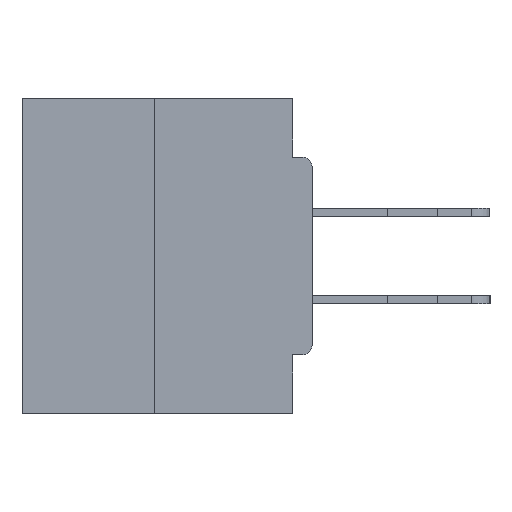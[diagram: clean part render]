
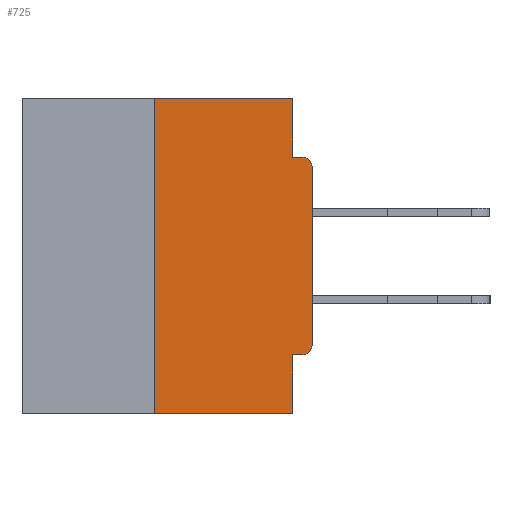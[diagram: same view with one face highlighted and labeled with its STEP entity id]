
A CAD part, left-side view. The second image highlights one B-rep face of the part: STEP entity #725.
In plain terms, the highlighted planar face has unit normal (-1, 0, 0).
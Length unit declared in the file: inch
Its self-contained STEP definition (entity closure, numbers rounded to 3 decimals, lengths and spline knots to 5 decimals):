
#447 = VECTOR ( 'NONE', #496, 39.37008 ) ;
#496 = DIRECTION ( 'NONE',  ( 0., 0., -1. ) ) ;
#539 = DIRECTION ( 'NONE',  ( 0., 0., 1. ) ) ;
#548 = VERTEX_POINT ( 'NONE', #23151 ) ;
#725 = ADVANCED_FACE ( 'NONE', ( #2220 ), #1923, .F. ) ;
#1036 = EDGE_CURVE ( 'NONE', #15112, #10786, #3096, .T. ) ;
#1923 = PLANE ( 'NONE',  #9730 ) ;
#2220 = FACE_OUTER_BOUND ( 'NONE', #24780, .T. ) ;
#2908 = DIRECTION ( 'NONE',  ( 0., -1., 0. ) ) ;
#3096 = LINE ( 'NONE', #11718, #33912 ) ;
#3262 = VECTOR ( 'NONE', #21967, 39.37008 ) ;
#4521 = EDGE_CURVE ( 'NONE', #15673, #548, #28752, .T. ) ;
#4667 = CARTESIAN_POINT ( 'NONE',  ( 0., 0.031, -0.4065 ) ) ;
#4798 = EDGE_CURVE ( 'NONE', #34067, #14897, #5996, .T. ) ;
#5551 = VECTOR ( 'NONE', #21708, 39.37008 ) ;
#5650 = ORIENTED_EDGE ( 'NONE', *, *, #13877, .F. ) ;
#5996 = LINE ( 'NONE', #7687, #3262 ) ;
#6161 = ORIENTED_EDGE ( 'NONE', *, *, #33916, .F. ) ;
#6210 = ORIENTED_EDGE ( 'NONE', *, *, #18368, .F. ) ;
#7275 = ORIENTED_EDGE ( 'NONE', *, *, #35363, .F. ) ;
#7687 = CARTESIAN_POINT ( 'NONE',  ( 0., 0.46, -0.5 ) ) ;
#7751 = CARTESIAN_POINT ( 'NONE',  ( 0., 0.015, -0.3915 ) ) ;
#8391 = DIRECTION ( 'NONE',  ( 0., -1., 0. ) ) ;
#9598 = VECTOR ( 'NONE', #8391, 39.37008 ) ;
#9730 = AXIS2_PLACEMENT_3D ( 'NONE', #25225, #10691, #13541 ) ;
#9937 = ORIENTED_EDGE ( 'NONE', *, *, #28549, .F. ) ;
#10206 = ORIENTED_EDGE ( 'NONE', *, *, #1036, .T. ) ;
#10496 = DIRECTION ( 'NONE',  ( -1., 0., 0. ) ) ;
#10594 = VERTEX_POINT ( 'NONE', #4667 ) ;
#10691 = DIRECTION ( 'NONE',  ( 1., 0., 0. ) ) ;
#10786 = VERTEX_POINT ( 'NONE', #31296 ) ;
#11718 = CARTESIAN_POINT ( 'NONE',  ( 0., 0., 0. ) ) ;
#12699 = ORIENTED_EDGE ( 'NONE', *, *, #4798, .T. ) ;
#13541 = DIRECTION ( 'NONE',  ( 0., 0., -1. ) ) ;
#13877 = EDGE_CURVE ( 'NONE', #34067, #15673, #26328, .T. ) ;
#14107 = CARTESIAN_POINT ( 'NONE',  ( 0., 0.25, -0.5 ) ) ;
#14121 = CARTESIAN_POINT ( 'NONE',  ( 0., 0., -0.3915 ) ) ;
#14760 = CARTESIAN_POINT ( 'NONE',  ( 0., 0.031, 0. ) ) ;
#14779 = LINE ( 'NONE', #14760, #447 ) ;
#14897 = VERTEX_POINT ( 'NONE', #21918 ) ;
#15112 = VERTEX_POINT ( 'NONE', #14121 ) ;
#15673 = VERTEX_POINT ( 'NONE', #30981 ) ;
#16180 = DIRECTION ( 'NONE',  ( 0., 0., -1. ) ) ;
#17092 = VERTEX_POINT ( 'NONE', #29850 ) ;
#18368 = EDGE_CURVE ( 'NONE', #23306, #10594, #19851, .T. ) ;
#18485 = EDGE_CURVE ( 'NONE', #10786, #21954, #35592, .T. ) ;
#19687 = CARTESIAN_POINT ( 'NONE',  ( 0., 0.46, 0. ) ) ;
#19851 = LINE ( 'NONE', #35964, #22055 ) ;
#20266 = CARTESIAN_POINT ( 'NONE',  ( 0., 0.25, 0. ) ) ;
#21588 = CARTESIAN_POINT ( 'NONE',  ( 0., 0.031, -0.5 ) ) ;
#21708 = DIRECTION ( 'NONE',  ( 0., 0., -1. ) ) ;
#21918 = CARTESIAN_POINT ( 'NONE',  ( 0., 0.031, -0.5 ) ) ;
#21954 = VERTEX_POINT ( 'NONE', #34400 ) ;
#21967 = DIRECTION ( 'NONE',  ( 0., -1., 0. ) ) ;
#22055 = VECTOR ( 'NONE', #27517, 39.37008 ) ;
#23100 = CARTESIAN_POINT ( 'NONE',  ( 0., 0., -0.0935 ) ) ;
#23151 = CARTESIAN_POINT ( 'NONE',  ( 0., 0.031, 0. ) ) ;
#23291 = AXIS2_PLACEMENT_3D ( 'NONE', #25122, #30874, #28133 ) ;
#23306 = VERTEX_POINT ( 'NONE', #32962 ) ;
#24536 = AXIS2_PLACEMENT_3D ( 'NONE', #7751, #10496, #16180 ) ;
#24547 = VECTOR ( 'NONE', #2908, 39.37008 ) ;
#24664 = ORIENTED_EDGE ( 'NONE', *, *, #18485, .T. ) ;
#24780 = EDGE_LOOP ( 'NONE', ( #35297, #5650, #12699, #6161, #6210, #34551, #10206, #24664, #7275, #9937 ) ) ;
#25122 = CARTESIAN_POINT ( 'NONE',  ( 0., 0.015, -0.1085 ) ) ;
#25225 = CARTESIAN_POINT ( 'NONE',  ( 0., 0.46, 0. ) ) ;
#26328 = LINE ( 'NONE', #20266, #31246 ) ;
#27517 = DIRECTION ( 'NONE',  ( 0., 1., 0. ) ) ;
#28133 = DIRECTION ( 'NONE',  ( 0., 0., -1. ) ) ;
#28549 = EDGE_CURVE ( 'NONE', #548, #17092, #14779, .T. ) ;
#28672 = DIRECTION ( 'NONE',  ( 0., 0., 1. ) ) ;
#28752 = LINE ( 'NONE', #19687, #9598 ) ;
#29624 = CIRCLE ( 'NONE', #24536, 0.015 ) ;
#29850 = CARTESIAN_POINT ( 'NONE',  ( 0., 0.031, -0.0935 ) ) ;
#29898 = LINE ( 'NONE', #23100, #24547 ) ;
#30874 = DIRECTION ( 'NONE',  ( -1., 0., 0. ) ) ;
#30981 = CARTESIAN_POINT ( 'NONE',  ( 0., 0.25, 0. ) ) ;
#31246 = VECTOR ( 'NONE', #539, 39.37008 ) ;
#31296 = CARTESIAN_POINT ( 'NONE',  ( 0., 0., -0.1085 ) ) ;
#32962 = CARTESIAN_POINT ( 'NONE',  ( 0., 0.015, -0.4065 ) ) ;
#33567 = EDGE_CURVE ( 'NONE', #23306, #15112, #29624, .T. ) ;
#33912 = VECTOR ( 'NONE', #28672, 39.37008 ) ;
#33916 = EDGE_CURVE ( 'NONE', #10594, #14897, #34556, .T. ) ;
#34067 = VERTEX_POINT ( 'NONE', #14107 ) ;
#34400 = CARTESIAN_POINT ( 'NONE',  ( 0., 0.015, -0.0935 ) ) ;
#34551 = ORIENTED_EDGE ( 'NONE', *, *, #33567, .T. ) ;
#34556 = LINE ( 'NONE', #21588, #5551 ) ;
#35297 = ORIENTED_EDGE ( 'NONE', *, *, #4521, .F. ) ;
#35363 = EDGE_CURVE ( 'NONE', #17092, #21954, #29898, .T. ) ;
#35592 = CIRCLE ( 'NONE', #23291, 0.015 ) ;
#35964 = CARTESIAN_POINT ( 'NONE',  ( 0., 0., -0.4065 ) ) ;
